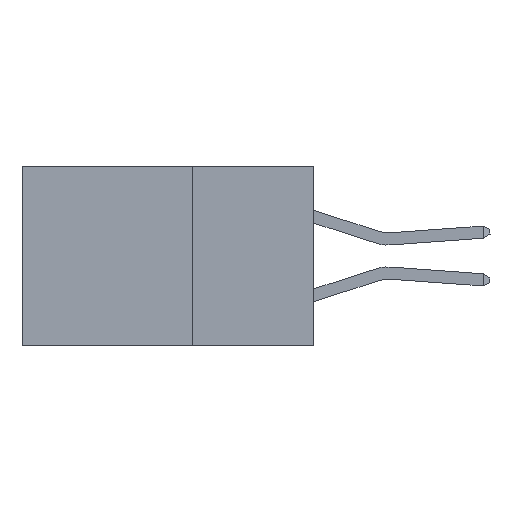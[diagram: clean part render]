
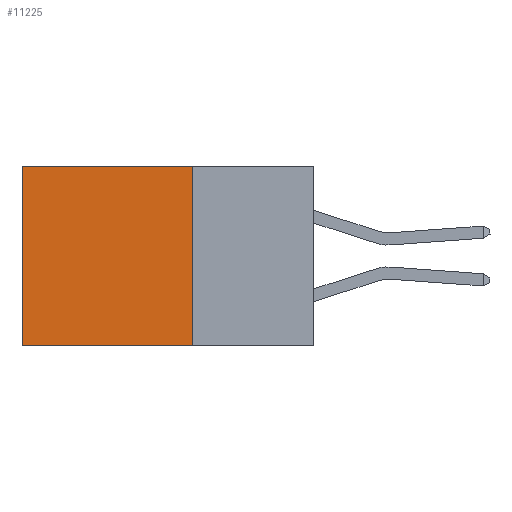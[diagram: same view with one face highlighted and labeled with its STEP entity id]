
A CAD part, left-side view. The second image highlights one B-rep face of the part: STEP entity #11225.
In plain terms, the highlighted planar face has unit normal (-1, 0, 0).
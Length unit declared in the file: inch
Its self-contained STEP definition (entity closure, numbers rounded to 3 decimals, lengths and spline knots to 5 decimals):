
#2275 = CARTESIAN_POINT ( 'NONE',  ( 0.2875, 0.6, 0. ) ) ;
#2576 = LINE ( 'NONE', #23747, #5035 ) ;
#3435 = DIRECTION ( 'NONE',  ( 0., 0., -1. ) ) ;
#3477 = EDGE_CURVE ( 'NONE', #15478, #10965, #12524, .T. ) ;
#5035 = VECTOR ( 'NONE', #6837, 39.37008 ) ;
#5045 = PLANE ( 'NONE',  #16863 ) ;
#6405 = DIRECTION ( 'NONE',  ( 0., 0., -1. ) ) ;
#6837 = DIRECTION ( 'NONE',  ( 0., 1., 0. ) ) ;
#7582 = EDGE_CURVE ( 'NONE', #12847, #21507, #17211, .T. ) ;
#8403 = ORIENTED_EDGE ( 'NONE', *, *, #17094, .F. ) ;
#9088 = VECTOR ( 'NONE', #6405, 39.37008 ) ;
#10537 = CARTESIAN_POINT ( 'NONE',  ( 0.2875, 0.25, 0. ) ) ;
#10965 = VERTEX_POINT ( 'NONE', #18551 ) ;
#11225 = ADVANCED_FACE ( 'NONE', ( #13033 ), #5045, .F. ) ;
#11572 = DIRECTION ( 'NONE',  ( 0., 0., -1. ) ) ;
#11927 = EDGE_CURVE ( 'NONE', #12847, #15478, #17945, .T. ) ;
#12006 = CARTESIAN_POINT ( 'NONE',  ( 0.2875, 0.25, -0.37 ) ) ;
#12047 = CARTESIAN_POINT ( 'NONE',  ( 0.2875, 0.25, 0. ) ) ;
#12524 = LINE ( 'NONE', #2275, #9088 ) ;
#12847 = VERTEX_POINT ( 'NONE', #10537 ) ;
#13033 = FACE_OUTER_BOUND ( 'NONE', #14647, .T. ) ;
#13817 = CARTESIAN_POINT ( 'NONE',  ( 0.2875, 0.25, 0. ) ) ;
#14647 = EDGE_LOOP ( 'NONE', ( #23313, #8403, #25825, #16725 ) ) ;
#15478 = VERTEX_POINT ( 'NONE', #20632 ) ;
#16330 = DIRECTION ( 'NONE',  ( 0., 1., 0. ) ) ;
#16352 = VECTOR ( 'NONE', #11572, 39.37008 ) ;
#16725 = ORIENTED_EDGE ( 'NONE', *, *, #11927, .T. ) ;
#16863 = AXIS2_PLACEMENT_3D ( 'NONE', #13817, #26106, #3435 ) ;
#17094 = EDGE_CURVE ( 'NONE', #21507, #10965, #2576, .T. ) ;
#17211 = LINE ( 'NONE', #23507, #16352 ) ;
#17812 = VECTOR ( 'NONE', #16330, 39.37008 ) ;
#17945 = LINE ( 'NONE', #12047, #17812 ) ;
#18551 = CARTESIAN_POINT ( 'NONE',  ( 0.2875, 0.6, -0.37 ) ) ;
#20632 = CARTESIAN_POINT ( 'NONE',  ( 0.2875, 0.6, 0. ) ) ;
#21507 = VERTEX_POINT ( 'NONE', #12006 ) ;
#23313 = ORIENTED_EDGE ( 'NONE', *, *, #3477, .T. ) ;
#23507 = CARTESIAN_POINT ( 'NONE',  ( 0.2875, 0.25, 0. ) ) ;
#23747 = CARTESIAN_POINT ( 'NONE',  ( 0.2875, 0.25, -0.37 ) ) ;
#25825 = ORIENTED_EDGE ( 'NONE', *, *, #7582, .F. ) ;
#26106 = DIRECTION ( 'NONE',  ( 1., 0., 0. ) ) ;
